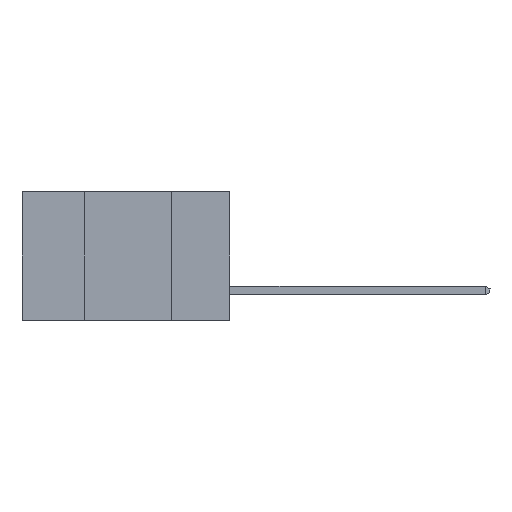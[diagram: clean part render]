
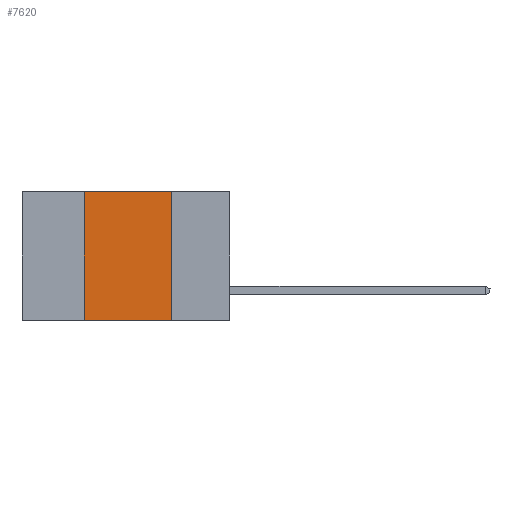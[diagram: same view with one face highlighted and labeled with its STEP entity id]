
A CAD part, left-side view. The second image highlights one B-rep face of the part: STEP entity #7620.
In plain terms, the highlighted planar face has unit normal (-1, 0, 0).
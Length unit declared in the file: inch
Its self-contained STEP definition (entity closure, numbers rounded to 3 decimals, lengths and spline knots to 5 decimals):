
#32 = ORIENTED_EDGE ( 'NONE', *, *, #9955, .T. ) ;
#131 = CARTESIAN_POINT ( 'NONE',  ( 0., 0.42, 0. ) ) ;
#655 = FACE_OUTER_BOUND ( 'NONE', #12526, .T. ) ;
#665 = DIRECTION ( 'NONE',  ( 0., 0., -1. ) ) ;
#790 = CARTESIAN_POINT ( 'NONE',  ( 0., 0.6, 0. ) ) ;
#1192 = CARTESIAN_POINT ( 'NONE',  ( 0., 0.42, -0.37 ) ) ;
#1921 = VERTEX_POINT ( 'NONE', #131 ) ;
#2107 = VECTOR ( 'NONE', #6484, 39.37008 ) ;
#2385 = VERTEX_POINT ( 'NONE', #8485 ) ;
#2537 = ORIENTED_EDGE ( 'NONE', *, *, #10825, .F. ) ;
#2900 = CARTESIAN_POINT ( 'NONE',  ( 0., 0.17, 0. ) ) ;
#4775 = LINE ( 'NONE', #11091, #9388 ) ;
#4857 = LINE ( 'NONE', #9932, #5255 ) ;
#4920 = DIRECTION ( 'NONE',  ( 1., 0., 0. ) ) ;
#4999 = EDGE_CURVE ( 'NONE', #9605, #1921, #12760, .T. ) ;
#5255 = VECTOR ( 'NONE', #665, 39.37008 ) ;
#6484 = DIRECTION ( 'NONE',  ( 0., 0., 1. ) ) ;
#7081 = VERTEX_POINT ( 'NONE', #2900 ) ;
#7586 = EDGE_CURVE ( 'NONE', #1921, #7081, #4775, .T. ) ;
#7620 = ADVANCED_FACE ( 'NONE', ( #655 ), #7999, .F. ) ;
#7909 = LINE ( 'NONE', #8985, #12268 ) ;
#7999 = PLANE ( 'NONE',  #8087 ) ;
#8087 = AXIS2_PLACEMENT_3D ( 'NONE', #790, #4920, #9993 ) ;
#8485 = CARTESIAN_POINT ( 'NONE',  ( 0., 0.17, -0.37 ) ) ;
#8885 = DIRECTION ( 'NONE',  ( 0., -1., 0. ) ) ;
#8985 = CARTESIAN_POINT ( 'NONE',  ( 0., 0.6, -0.37 ) ) ;
#9112 = ORIENTED_EDGE ( 'NONE', *, *, #7586, .F. ) ;
#9388 = VECTOR ( 'NONE', #8885, 39.37008 ) ;
#9605 = VERTEX_POINT ( 'NONE', #11570 ) ;
#9747 = ORIENTED_EDGE ( 'NONE', *, *, #4999, .F. ) ;
#9932 = CARTESIAN_POINT ( 'NONE',  ( 0., 0.17, -0.37 ) ) ;
#9955 = EDGE_CURVE ( 'NONE', #9605, #2385, #7909, .T. ) ;
#9993 = DIRECTION ( 'NONE',  ( 0., 0., -1. ) ) ;
#10825 = EDGE_CURVE ( 'NONE', #7081, #2385, #4857, .T. ) ;
#10990 = DIRECTION ( 'NONE',  ( 0., -1., 0. ) ) ;
#11091 = CARTESIAN_POINT ( 'NONE',  ( 0., 0.6, 0. ) ) ;
#11570 = CARTESIAN_POINT ( 'NONE',  ( 0., 0.42, -0.37 ) ) ;
#12268 = VECTOR ( 'NONE', #10990, 39.37008 ) ;
#12526 = EDGE_LOOP ( 'NONE', ( #2537, #9112, #9747, #32 ) ) ;
#12760 = LINE ( 'NONE', #1192, #2107 ) ;
